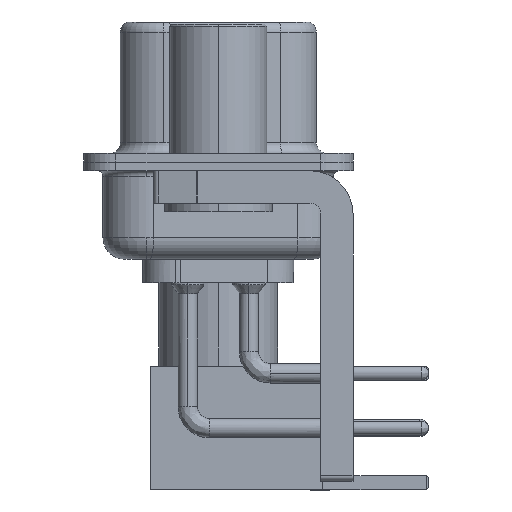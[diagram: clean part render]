
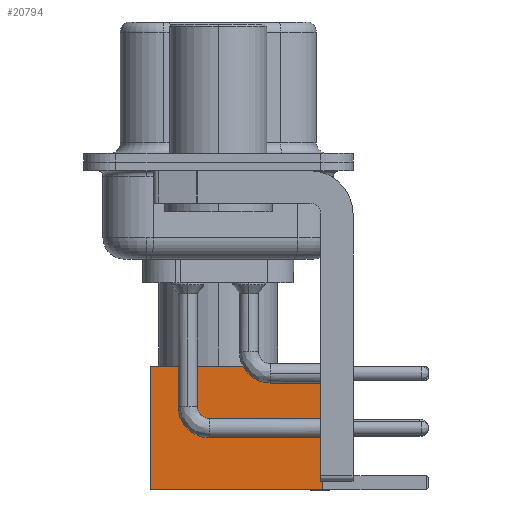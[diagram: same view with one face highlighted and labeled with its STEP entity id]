
A CAD part, left-side view. The second image highlights one B-rep face of the part: STEP entity #20794.
In plain terms, the highlighted face is planar.
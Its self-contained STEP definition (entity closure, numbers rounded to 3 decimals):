
#1039 = ORIENTED_EDGE ( 'NONE', *, *, #2267, .F. ) ;
#1318 = DIRECTION ( 'NONE',  ( 0., 1., 0. ) ) ;
#2267 = EDGE_CURVE ( 'NONE', #12468, #6518, #25605, .T. ) ;
#3470 = AXIS2_PLACEMENT_3D ( 'NONE', #17387, #1318, #22875 ) ;
#5067 = EDGE_CURVE ( 'NONE', #21691, #10737, #11470, .T. ) ;
#5410 = ORIENTED_EDGE ( 'NONE', *, *, #10178, .T. ) ;
#6518 = VERTEX_POINT ( 'NONE', #14113 ) ;
#7543 = CARTESIAN_POINT ( 'NONE',  ( 0., 2.875, 0. ) ) ;
#7624 = CARTESIAN_POINT ( 'NONE',  ( 2.875, 2.875, 8. ) ) ;
#9320 = VECTOR ( 'NONE', #13721, 1000. ) ;
#10178 = EDGE_CURVE ( 'NONE', #12468, #21691, #10933, .T. ) ;
#10737 = VERTEX_POINT ( 'NONE', #14946 ) ;
#10933 = LINE ( 'NONE', #18879, #14279 ) ;
#11470 = LINE ( 'NONE', #7543, #22468 ) ;
#11560 = CARTESIAN_POINT ( 'NONE',  ( -2.875, 2.875, 0. ) ) ;
#12468 = VERTEX_POINT ( 'NONE', #7624 ) ;
#13591 = EDGE_LOOP ( 'NONE', ( #5410, #23425, #14637, #1039 ) ) ;
#13721 = DIRECTION ( 'NONE',  ( -1., 0., 0. ) ) ;
#14113 = CARTESIAN_POINT ( 'NONE',  ( -2.875, 2.875, 8. ) ) ;
#14279 = VECTOR ( 'NONE', #22938, 1000. ) ;
#14637 = ORIENTED_EDGE ( 'NONE', *, *, #25391, .F. ) ;
#14946 = CARTESIAN_POINT ( 'NONE',  ( -2.875, 2.875, 0. ) ) ;
#15297 = PLANE ( 'NONE',  #3470 ) ;
#15499 = DIRECTION ( 'NONE',  ( -1., 0., 0. ) ) ;
#15662 = CARTESIAN_POINT ( 'NONE',  ( 0., 2.875, 8. ) ) ;
#17387 = CARTESIAN_POINT ( 'NONE',  ( 2.875, 2.875, 0. ) ) ;
#18879 = CARTESIAN_POINT ( 'NONE',  ( 2.875, 2.875, 0. ) ) ;
#19071 = FACE_OUTER_BOUND ( 'NONE', #13591, .T. ) ;
#19959 = CARTESIAN_POINT ( 'NONE',  ( 2.875, 2.875, 0. ) ) ;
#20794 = ADVANCED_FACE ( 'NONE', ( #19071 ), #15297, .T. ) ;
#21691 = VERTEX_POINT ( 'NONE', #19959 ) ;
#21861 = LINE ( 'NONE', #11560, #23176 ) ;
#22468 = VECTOR ( 'NONE', #15499, 1000. ) ;
#22875 = DIRECTION ( 'NONE',  ( 0., 0., 1. ) ) ;
#22938 = DIRECTION ( 'NONE',  ( 0., 0., -1. ) ) ;
#23176 = VECTOR ( 'NONE', #25787, 1000. ) ;
#23425 = ORIENTED_EDGE ( 'NONE', *, *, #5067, .T. ) ;
#25391 = EDGE_CURVE ( 'NONE', #6518, #10737, #21861, .T. ) ;
#25605 = LINE ( 'NONE', #15662, #9320 ) ;
#25787 = DIRECTION ( 'NONE',  ( 0., 0., -1. ) ) ;
